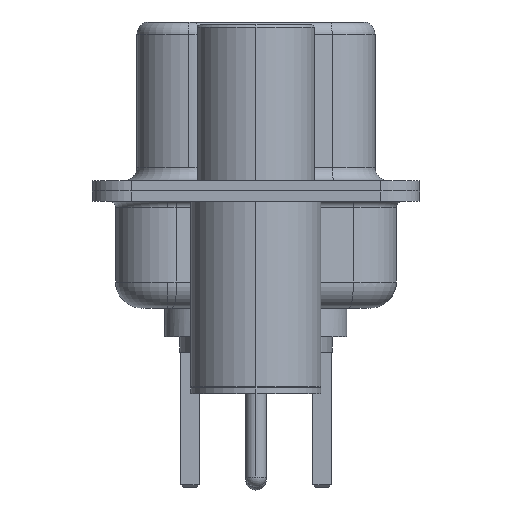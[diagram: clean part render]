
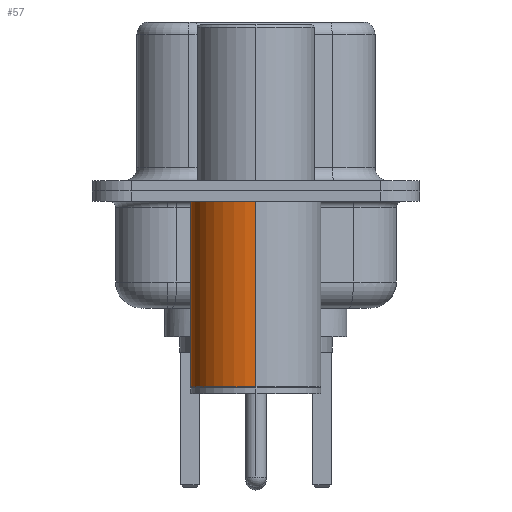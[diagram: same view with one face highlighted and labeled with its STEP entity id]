
A CAD part, left-side view. The second image highlights one B-rep face of the part: STEP entity #57.
In plain terms, the highlighted cylindrical face has radius 2.5 mm (diameter 5 mm), a partial arc.
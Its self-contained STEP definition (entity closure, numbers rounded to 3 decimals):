
#57 = ADVANCED_FACE ( 'NONE', ( #3054 ), #15761, .T. ) ;
#263 = VERTEX_POINT ( 'NONE', #12879 ) ;
#296 = EDGE_CURVE ( 'NONE', #263, #17135, #12122, .T. ) ;
#844 = DIRECTION ( 'NONE',  ( 1., 0., 0. ) ) ;
#1104 = AXIS2_PLACEMENT_3D ( 'NONE', #1848, #13422, #3497 ) ;
#1228 = CARTESIAN_POINT ( 'NONE',  ( -2.5, 0., -0.4 ) ) ;
#1848 = CARTESIAN_POINT ( 'NONE',  ( 0., 0., -0.4 ) ) ;
#1864 = CIRCLE ( 'NONE', #1104, 2.5 ) ;
#2398 = ORIENTED_EDGE ( 'NONE', *, *, #14109, .T. ) ;
#3054 = FACE_OUTER_BOUND ( 'NONE', #9026, .T. ) ;
#3497 = DIRECTION ( 'NONE',  ( 1., 0., 0. ) ) ;
#3677 = LINE ( 'NONE', #13661, #8636 ) ;
#3747 = DIRECTION ( 'NONE',  ( 0., 0., 1. ) ) ;
#4144 = EDGE_CURVE ( 'NONE', #17135, #12924, #1864, .T. ) ;
#4749 = CARTESIAN_POINT ( 'NONE',  ( -2.5, 0., -7.525 ) ) ;
#5170 = CARTESIAN_POINT ( 'NONE',  ( 2.5, 0., -0.4 ) ) ;
#7575 = CARTESIAN_POINT ( 'NONE',  ( 0., 0., -7.525 ) ) ;
#7734 = VECTOR ( 'NONE', #14543, 1000. ) ;
#8636 = VECTOR ( 'NONE', #3747, 1000. ) ;
#9026 = EDGE_LOOP ( 'NONE', ( #2398, #14708, #21061, #15228 ) ) ;
#9224 = DIRECTION ( 'NONE',  ( 1., 0., 0. ) ) ;
#10248 = EDGE_CURVE ( 'NONE', #11838, #12924, #3677, .T. ) ;
#11838 = VERTEX_POINT ( 'NONE', #4749 ) ;
#12122 = LINE ( 'NONE', #14761, #7734 ) ;
#12416 = AXIS2_PLACEMENT_3D ( 'NONE', #21226, #16353, #844 ) ;
#12879 = CARTESIAN_POINT ( 'NONE',  ( 2.5, 0., -7.525 ) ) ;
#12924 = VERTEX_POINT ( 'NONE', #1228 ) ;
#13422 = DIRECTION ( 'NONE',  ( 0., 0., 1. ) ) ;
#13661 = CARTESIAN_POINT ( 'NONE',  ( -2.5, 0., 0.581 ) ) ;
#14109 = EDGE_CURVE ( 'NONE', #263, #11838, #15067, .T. ) ;
#14543 = DIRECTION ( 'NONE',  ( 0., 0., 1. ) ) ;
#14708 = ORIENTED_EDGE ( 'NONE', *, *, #10248, .T. ) ;
#14761 = CARTESIAN_POINT ( 'NONE',  ( 2.5, 0., 0.581 ) ) ;
#15067 = CIRCLE ( 'NONE', #20112, 2.5 ) ;
#15228 = ORIENTED_EDGE ( 'NONE', *, *, #296, .F. ) ;
#15761 = CYLINDRICAL_SURFACE ( 'NONE', #12416, 2.5 ) ;
#16353 = DIRECTION ( 'NONE',  ( 0., 0., 1. ) ) ;
#17135 = VERTEX_POINT ( 'NONE', #5170 ) ;
#19156 = DIRECTION ( 'NONE',  ( 0., 0., 1. ) ) ;
#20112 = AXIS2_PLACEMENT_3D ( 'NONE', #7575, #19156, #9224 ) ;
#21061 = ORIENTED_EDGE ( 'NONE', *, *, #4144, .F. ) ;
#21226 = CARTESIAN_POINT ( 'NONE',  ( 0., 0., 0.581 ) ) ;
